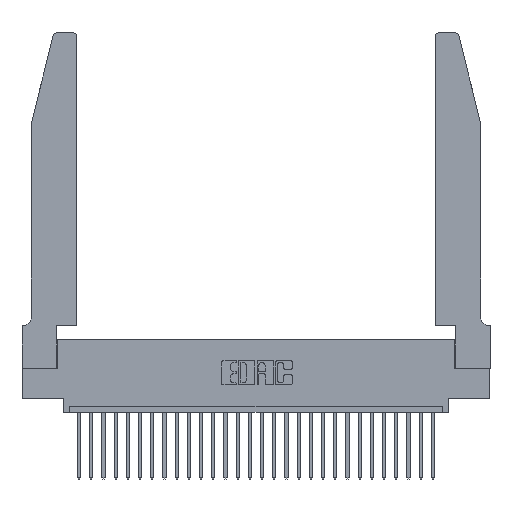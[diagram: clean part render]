
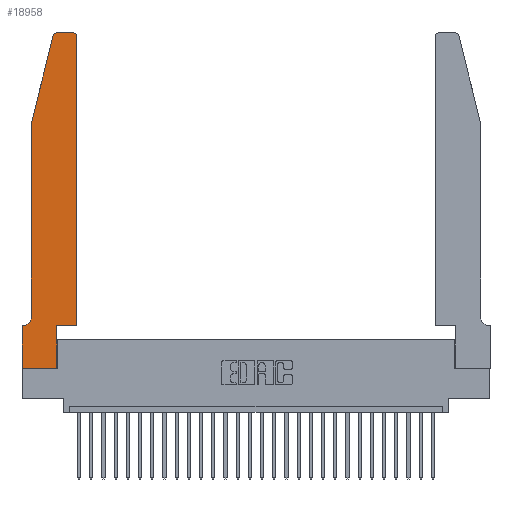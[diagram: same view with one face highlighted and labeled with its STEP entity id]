
A CAD part, top view. The second image highlights one B-rep face of the part: STEP entity #18958.
In plain terms, the highlighted planar face has unit normal (0, 0, 1).
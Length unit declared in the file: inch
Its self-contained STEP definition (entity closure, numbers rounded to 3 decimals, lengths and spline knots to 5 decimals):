
#129 = CARTESIAN_POINT ( 'NONE',  ( 0.0755, 0.42, 0.37 ) ) ;
#677 = LINE ( 'NONE', #22368, #5966 ) ;
#715 = DIRECTION ( 'NONE',  ( 0., 0., 1. ) ) ;
#993 = FACE_OUTER_BOUND ( 'NONE', #24931, .T. ) ;
#1056 = VERTEX_POINT ( 'NONE', #4604 ) ;
#1289 = ORIENTED_EDGE ( 'NONE', *, *, #25013, .T. ) ;
#1621 = LINE ( 'NONE', #11985, #4421 ) ;
#1764 = EDGE_CURVE ( 'NONE', #25821, #9672, #25546, .T. ) ;
#1775 = CARTESIAN_POINT ( 'NONE',  ( 0., 0.35, 0.37 ) ) ;
#2414 = AXIS2_PLACEMENT_3D ( 'NONE', #14231, #715, #5007 ) ;
#2485 = LINE ( 'NONE', #5278, #6049 ) ;
#2744 = DIRECTION ( 'NONE',  ( -1., 0., 0. ) ) ;
#3190 = DIRECTION ( 'NONE',  ( 0., 1., 0. ) ) ;
#3952 = AXIS2_PLACEMENT_3D ( 'NONE', #1775, #28163, #28568 ) ;
#4076 = ORIENTED_EDGE ( 'NONE', *, *, #1764, .T. ) ;
#4129 = VECTOR ( 'NONE', #5692, 39.37008 ) ;
#4421 = VECTOR ( 'NONE', #5054, 39.37008 ) ;
#4604 = CARTESIAN_POINT ( 'NONE',  ( 0.0055, 0.35, 0.37 ) ) ;
#4699 = ORIENTED_EDGE ( 'NONE', *, *, #7694, .T. ) ;
#5007 = DIRECTION ( 'NONE',  ( 1., 0., 0. ) ) ;
#5054 = DIRECTION ( 'NONE',  ( -0.239, -0.971, 0. ) ) ;
#5278 = CARTESIAN_POINT ( 'NONE',  ( 0., 0., 0.37 ) ) ;
#5692 = DIRECTION ( 'NONE',  ( 1., 0., 0. ) ) ;
#5847 = ORIENTED_EDGE ( 'NONE', *, *, #16567, .T. ) ;
#5966 = VECTOR ( 'NONE', #22455, 39.37008 ) ;
#6049 = VECTOR ( 'NONE', #9854, 39.37008 ) ;
#6256 = CIRCLE ( 'NONE', #2414, 0.03 ) ;
#6723 = ORIENTED_EDGE ( 'NONE', *, *, #15609, .T. ) ;
#6946 = CARTESIAN_POINT ( 'NONE',  ( 0.4505, 0.35, 0.37 ) ) ;
#7043 = CARTESIAN_POINT ( 'NONE',  ( 0.0055, 0.42, 0.37 ) ) ;
#7694 = EDGE_CURVE ( 'NONE', #14683, #25821, #1621, .T. ) ;
#7887 = VERTEX_POINT ( 'NONE', #23221 ) ;
#8604 = EDGE_CURVE ( 'NONE', #23467, #21218, #2485, .T. ) ;
#9270 = LINE ( 'NONE', #17742, #27180 ) ;
#9672 = VERTEX_POINT ( 'NONE', #129 ) ;
#9854 = DIRECTION ( 'NONE',  ( 0., -1., 0. ) ) ;
#10093 = ORIENTED_EDGE ( 'NONE', *, *, #8604, .T. ) ;
#11353 = EDGE_CURVE ( 'NONE', #7887, #13536, #6256, .T. ) ;
#11365 = VECTOR ( 'NONE', #25984, 39.37008 ) ;
#11858 = CARTESIAN_POINT ( 'NONE',  ( 0.0755, 2., 0.37 ) ) ;
#11985 = CARTESIAN_POINT ( 'NONE',  ( 0.0755, 2., 0.37 ) ) ;
#12426 = LINE ( 'NONE', #16286, #26112 ) ;
#12613 = DIRECTION ( 'NONE',  ( 0., 0., 1. ) ) ;
#12807 = LINE ( 'NONE', #17271, #11365 ) ;
#13406 = DIRECTION ( 'NONE',  ( 1., 0., 0. ) ) ;
#13536 = VERTEX_POINT ( 'NONE', #25689 ) ;
#14231 = CARTESIAN_POINT ( 'NONE',  ( 0.4205, 2.72, 0.37 ) ) ;
#14649 = CIRCLE ( 'NONE', #15383, 0.07 ) ;
#14683 = VERTEX_POINT ( 'NONE', #21873 ) ;
#14930 = CARTESIAN_POINT ( 'NONE',  ( 0.2865, 0.35, 0.37 ) ) ;
#15383 = AXIS2_PLACEMENT_3D ( 'NONE', #7043, #22615, #24850 ) ;
#15609 = EDGE_CURVE ( 'NONE', #17966, #18719, #9270, .T. ) ;
#16286 = CARTESIAN_POINT ( 'NONE',  ( 0.2605, 2.75, 0.37 ) ) ;
#16500 = LINE ( 'NONE', #16953, #4129 ) ;
#16505 = CARTESIAN_POINT ( 'NONE',  ( 0.0755, 0.35, 0.37 ) ) ;
#16567 = EDGE_CURVE ( 'NONE', #13536, #25110, #12426, .T. ) ;
#16953 = CARTESIAN_POINT ( 'NONE',  ( 0.4505, 0.35, 0.37 ) ) ;
#17160 = VECTOR ( 'NONE', #27267, 39.37008 ) ;
#17185 = CARTESIAN_POINT ( 'NONE',  ( 0., 0.35, 0.37 ) ) ;
#17271 = CARTESIAN_POINT ( 'NONE',  ( 0.4505, 0.35, 0.37 ) ) ;
#17520 = ORIENTED_EDGE ( 'NONE', *, *, #28156, .T. ) ;
#17742 = CARTESIAN_POINT ( 'NONE',  ( 0.2865, 0.35, 0.37 ) ) ;
#17794 = ORIENTED_EDGE ( 'NONE', *, *, #24551, .T. ) ;
#17966 = VERTEX_POINT ( 'NONE', #25404 ) ;
#18379 = AXIS2_PLACEMENT_3D ( 'NONE', #23814, #12613, #13406 ) ;
#18655 = DIRECTION ( 'NONE',  ( -1., 0., 0. ) ) ;
#18719 = VERTEX_POINT ( 'NONE', #14930 ) ;
#18958 = ADVANCED_FACE ( 'NONE', ( #993 ), #19774, .T. ) ;
#19774 = PLANE ( 'NONE',  #3952 ) ;
#19838 = CARTESIAN_POINT ( 'NONE',  ( 0.0755, 2., 0.37 ) ) ;
#21216 = VERTEX_POINT ( 'NONE', #6946 ) ;
#21218 = VERTEX_POINT ( 'NONE', #27286 ) ;
#21232 = EDGE_CURVE ( 'NONE', #9672, #1056, #14649, .T. ) ;
#21873 = CARTESIAN_POINT ( 'NONE',  ( 0.25487, 2.72718, 0.37 ) ) ;
#22368 = CARTESIAN_POINT ( 'NONE',  ( 0., 0., 0.37 ) ) ;
#22455 = DIRECTION ( 'NONE',  ( 1., 0., 0. ) ) ;
#22615 = DIRECTION ( 'NONE',  ( 0., 0., -1. ) ) ;
#23033 = EDGE_CURVE ( 'NONE', #25110, #14683, #25739, .T. ) ;
#23150 = EDGE_CURVE ( 'NONE', #1056, #23467, #25395, .T. ) ;
#23221 = CARTESIAN_POINT ( 'NONE',  ( 0.4505, 2.72, 0.37 ) ) ;
#23301 = VECTOR ( 'NONE', #18655, 39.37008 ) ;
#23467 = VERTEX_POINT ( 'NONE', #17185 ) ;
#23814 = CARTESIAN_POINT ( 'NONE',  ( 0.284, 2.72, 0.37 ) ) ;
#24551 = EDGE_CURVE ( 'NONE', #21218, #17966, #677, .T. ) ;
#24581 = CARTESIAN_POINT ( 'NONE',  ( 0.284, 2.75, 0.37 ) ) ;
#24748 = ORIENTED_EDGE ( 'NONE', *, *, #11353, .T. ) ;
#24850 = DIRECTION ( 'NONE',  ( -1., 0., 0. ) ) ;
#24931 = EDGE_LOOP ( 'NONE', ( #5847, #26476, #4699, #4076, #27383, #27941, #10093, #17794, #6723, #1289, #17520, #24748 ) ) ;
#25013 = EDGE_CURVE ( 'NONE', #18719, #21216, #16500, .T. ) ;
#25110 = VERTEX_POINT ( 'NONE', #24581 ) ;
#25395 = LINE ( 'NONE', #16505, #23301 ) ;
#25404 = CARTESIAN_POINT ( 'NONE',  ( 0.2865, 0., 0.37 ) ) ;
#25546 = LINE ( 'NONE', #11858, #17160 ) ;
#25689 = CARTESIAN_POINT ( 'NONE',  ( 0.4205, 2.75, 0.37 ) ) ;
#25739 = CIRCLE ( 'NONE', #18379, 0.03 ) ;
#25821 = VERTEX_POINT ( 'NONE', #19838 ) ;
#25984 = DIRECTION ( 'NONE',  ( 0., 1., 0. ) ) ;
#26112 = VECTOR ( 'NONE', #2744, 39.37008 ) ;
#26476 = ORIENTED_EDGE ( 'NONE', *, *, #23033, .T. ) ;
#27180 = VECTOR ( 'NONE', #3190, 39.37008 ) ;
#27267 = DIRECTION ( 'NONE',  ( 0., -1., 0. ) ) ;
#27286 = CARTESIAN_POINT ( 'NONE',  ( 0., 0., 0.37 ) ) ;
#27383 = ORIENTED_EDGE ( 'NONE', *, *, #21232, .T. ) ;
#27941 = ORIENTED_EDGE ( 'NONE', *, *, #23150, .T. ) ;
#28156 = EDGE_CURVE ( 'NONE', #21216, #7887, #12807, .T. ) ;
#28163 = DIRECTION ( 'NONE',  ( 0., 0., 1. ) ) ;
#28568 = DIRECTION ( 'NONE',  ( 1., 0., 0. ) ) ;
